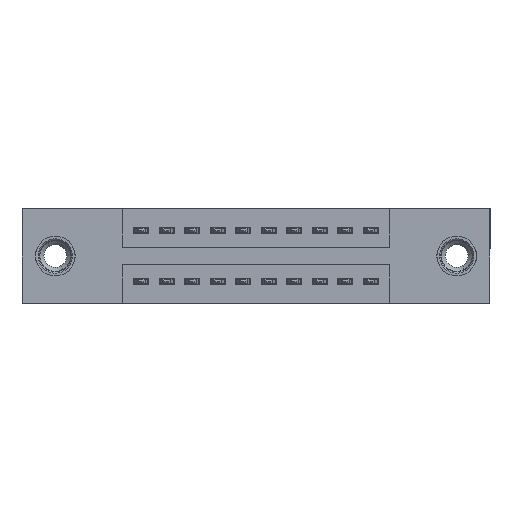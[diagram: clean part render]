
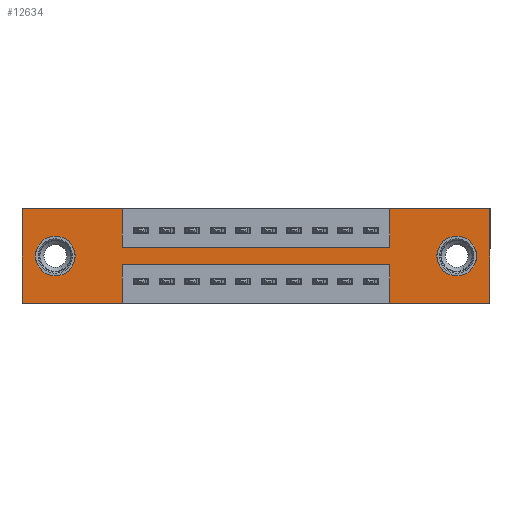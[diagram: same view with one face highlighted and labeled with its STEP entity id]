
A CAD part, front view. The second image highlights one B-rep face of the part: STEP entity #12634.
In plain terms, the highlighted planar face has unit normal (0, -1, 0).
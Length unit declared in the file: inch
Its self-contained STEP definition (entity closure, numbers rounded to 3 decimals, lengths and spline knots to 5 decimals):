
#121 = CARTESIAN_POINT ( 'NONE',  ( 0., 0., 0. ) ) ;
#182 = ORIENTED_EDGE ( 'NONE', *, *, #13849, .F. ) ;
#224 = CARTESIAN_POINT ( 'NONE',  ( 1.705, 0., -0.263 ) ) ;
#312 = LINE ( 'NONE', #5380, #14048 ) ;
#617 = EDGE_CURVE ( 'NONE', #8967, #3346, #3649, .T. ) ;
#716 = CIRCLE ( 'NONE', #15169, 0.078 ) ;
#773 = CARTESIAN_POINT ( 'NONE',  ( 0., 0., -0.37 ) ) ;
#866 = EDGE_CURVE ( 'NONE', #4796, #4143, #10822, .T. ) ;
#882 = DIRECTION ( 'NONE',  ( 1., 0., 0. ) ) ;
#990 = EDGE_CURVE ( 'NONE', #4143, #8967, #6941, .T. ) ;
#1279 = CARTESIAN_POINT ( 'NONE',  ( 0.3925, 0., 0. ) ) ;
#1297 = CARTESIAN_POINT ( 'NONE',  ( 0.3925, 0., -0.37 ) ) ;
#1778 = CARTESIAN_POINT ( 'NONE',  ( 1.4425, 0., -0.15 ) ) ;
#1867 = ORIENTED_EDGE ( 'NONE', *, *, #10916, .F. ) ;
#1991 = VERTEX_POINT ( 'NONE', #10762 ) ;
#1994 = DIRECTION ( 'NONE',  ( 0., 0., 1. ) ) ;
#2350 = CARTESIAN_POINT ( 'NONE',  ( 1.705, 0., -0.185 ) ) ;
#2549 = VERTEX_POINT ( 'NONE', #1279 ) ;
#2625 = CARTESIAN_POINT ( 'NONE',  ( 0., 0., 0. ) ) ;
#2673 = EDGE_CURVE ( 'NONE', #3155, #16917, #12116, .T. ) ;
#2813 = AXIS2_PLACEMENT_3D ( 'NONE', #13764, #5998, #15003 ) ;
#2911 = CIRCLE ( 'NONE', #12442, 0.078 ) ;
#3048 = CARTESIAN_POINT ( 'NONE',  ( 0.3925, 0., -0.22 ) ) ;
#3155 = VERTEX_POINT ( 'NONE', #12738 ) ;
#3212 = VECTOR ( 'NONE', #882, 39.37008 ) ;
#3346 = VERTEX_POINT ( 'NONE', #17023 ) ;
#3509 = CARTESIAN_POINT ( 'NONE',  ( 0.3925, 0., -0.15 ) ) ;
#3550 = ORIENTED_EDGE ( 'NONE', *, *, #15050, .F. ) ;
#3649 = LINE ( 'NONE', #121, #3212 ) ;
#3744 = CARTESIAN_POINT ( 'NONE',  ( 1.4425, 0., 0. ) ) ;
#3750 = DIRECTION ( 'NONE',  ( 0., 0., -1. ) ) ;
#3848 = VECTOR ( 'NONE', #6749, 39.37008 ) ;
#3890 = DIRECTION ( 'NONE',  ( 0., 0., 1. ) ) ;
#4140 = DIRECTION ( 'NONE',  ( 1., 0., 0. ) ) ;
#4143 = VERTEX_POINT ( 'NONE', #1778 ) ;
#4450 = VECTOR ( 'NONE', #16016, 39.37008 ) ;
#4638 = CARTESIAN_POINT ( 'NONE',  ( 1.4425, 0., 0. ) ) ;
#4796 = VERTEX_POINT ( 'NONE', #13777 ) ;
#4904 = VERTEX_POINT ( 'NONE', #12872 ) ;
#5045 = EDGE_CURVE ( 'NONE', #2549, #4796, #312, .T. ) ;
#5380 = CARTESIAN_POINT ( 'NONE',  ( 0.3925, 0., 0. ) ) ;
#5567 = ORIENTED_EDGE ( 'NONE', *, *, #12594, .T. ) ;
#5739 = VECTOR ( 'NONE', #14583, 39.37008 ) ;
#5972 = VERTEX_POINT ( 'NONE', #13733 ) ;
#5981 = CARTESIAN_POINT ( 'NONE',  ( 0., 0., -0.37 ) ) ;
#5998 = DIRECTION ( 'NONE',  ( 0., 1., 0. ) ) ;
#6016 = CARTESIAN_POINT ( 'NONE',  ( 1.4425, 0., -0.37 ) ) ;
#6048 = DIRECTION ( 'NONE',  ( 0., -1., 0. ) ) ;
#6098 = CARTESIAN_POINT ( 'NONE',  ( 0.13, 0., -0.263 ) ) ;
#6144 = CARTESIAN_POINT ( 'NONE',  ( 1.835, 0., 0. ) ) ;
#6189 = EDGE_CURVE ( 'NONE', #14736, #5972, #7317, .T. ) ;
#6308 = EDGE_LOOP ( 'NONE', ( #6847, #15502, #182, #16227, #7313, #9297, #8801, #12452, #8938, #3550, #16236, #1867 ) ) ;
#6440 = FACE_BOUND ( 'NONE', #16244, .T. ) ;
#6448 = EDGE_CURVE ( 'NONE', #7576, #1991, #716, .T. ) ;
#6749 = DIRECTION ( 'NONE',  ( 0., 0., -1. ) ) ;
#6782 = LINE ( 'NONE', #11856, #16581 ) ;
#6847 = ORIENTED_EDGE ( 'NONE', *, *, #6189, .F. ) ;
#6941 = LINE ( 'NONE', #3744, #5739 ) ;
#7313 = ORIENTED_EDGE ( 'NONE', *, *, #16451, .F. ) ;
#7314 = EDGE_CURVE ( 'NONE', #13949, #8840, #8773, .T. ) ;
#7317 = LINE ( 'NONE', #1297, #3848 ) ;
#7379 = CARTESIAN_POINT ( 'NONE',  ( 1.705, 0., -0.185 ) ) ;
#7576 = VERTEX_POINT ( 'NONE', #224 ) ;
#7912 = DIRECTION ( 'NONE',  ( 0., 0., 1. ) ) ;
#8158 = AXIS2_PLACEMENT_3D ( 'NONE', #8648, #6048, #15055 ) ;
#8265 = LINE ( 'NONE', #6016, #15074 ) ;
#8354 = CARTESIAN_POINT ( 'NONE',  ( 1.835, 0., -0.37 ) ) ;
#8471 = EDGE_CURVE ( 'NONE', #1991, #7576, #2911, .T. ) ;
#8606 = DIRECTION ( 'NONE',  ( 0., 1., 0. ) ) ;
#8648 = CARTESIAN_POINT ( 'NONE',  ( 0., 0., -0.37 ) ) ;
#8740 = DIRECTION ( 'NONE',  ( 0., 0., -1. ) ) ;
#8773 = LINE ( 'NONE', #2625, #12170 ) ;
#8801 = ORIENTED_EDGE ( 'NONE', *, *, #990, .F. ) ;
#8816 = DIRECTION ( 'NONE',  ( 0., 0., -1. ) ) ;
#8838 = DIRECTION ( 'NONE',  ( -1., 0., 0. ) ) ;
#8840 = VERTEX_POINT ( 'NONE', #10787 ) ;
#8846 = VECTOR ( 'NONE', #8816, 39.37008 ) ;
#8932 = CARTESIAN_POINT ( 'NONE',  ( 0.13, 0., -0.185 ) ) ;
#8938 = ORIENTED_EDGE ( 'NONE', *, *, #5045, .F. ) ;
#8967 = VERTEX_POINT ( 'NONE', #4638 ) ;
#9252 = LINE ( 'NONE', #6144, #8846 ) ;
#9297 = ORIENTED_EDGE ( 'NONE', *, *, #617, .F. ) ;
#9544 = FACE_OUTER_BOUND ( 'NONE', #6308, .T. ) ;
#9771 = ORIENTED_EDGE ( 'NONE', *, *, #8471, .T. ) ;
#9969 = PLANE ( 'NONE',  #8158 ) ;
#10200 = LINE ( 'NONE', #15160, #16111 ) ;
#10440 = VECTOR ( 'NONE', #4140, 39.37008 ) ;
#10638 = DIRECTION ( 'NONE',  ( 1., 0., 0. ) ) ;
#10762 = CARTESIAN_POINT ( 'NONE',  ( 1.705, 0., -0.107 ) ) ;
#10787 = CARTESIAN_POINT ( 'NONE',  ( 0., 0., 0. ) ) ;
#10822 = LINE ( 'NONE', #3509, #10440 ) ;
#10835 = LINE ( 'NONE', #5981, #13466 ) ;
#10916 = EDGE_CURVE ( 'NONE', #5972, #13949, #10200, .T. ) ;
#11051 = CARTESIAN_POINT ( 'NONE',  ( 0.3925, 0., -0.22 ) ) ;
#11250 = CARTESIAN_POINT ( 'NONE',  ( 1.4425, 0., -0.37 ) ) ;
#11328 = EDGE_CURVE ( 'NONE', #4904, #14736, #14363, .T. ) ;
#11332 = AXIS2_PLACEMENT_3D ( 'NONE', #8932, #8606, #3890 ) ;
#11593 = DIRECTION ( 'NONE',  ( 0., 1., 0. ) ) ;
#11856 = CARTESIAN_POINT ( 'NONE',  ( 0., 0., 0. ) ) ;
#12116 = CIRCLE ( 'NONE', #11332, 0.078 ) ;
#12170 = VECTOR ( 'NONE', #7912, 39.37008 ) ;
#12442 = AXIS2_PLACEMENT_3D ( 'NONE', #2350, #11593, #3750 ) ;
#12452 = ORIENTED_EDGE ( 'NONE', *, *, #866, .F. ) ;
#12594 = EDGE_CURVE ( 'NONE', #16917, #3155, #16262, .T. ) ;
#12634 = ADVANCED_FACE ( 'NONE', ( #6440, #15870, #9544 ), #9969, .T. ) ;
#12738 = CARTESIAN_POINT ( 'NONE',  ( 0.13, 0., -0.107 ) ) ;
#12872 = CARTESIAN_POINT ( 'NONE',  ( 1.4425, 0., -0.22 ) ) ;
#13466 = VECTOR ( 'NONE', #14983, 39.37008 ) ;
#13597 = ORIENTED_EDGE ( 'NONE', *, *, #2673, .T. ) ;
#13733 = CARTESIAN_POINT ( 'NONE',  ( 0.3925, 0., -0.37 ) ) ;
#13764 = CARTESIAN_POINT ( 'NONE',  ( 0.13, 0., -0.185 ) ) ;
#13777 = CARTESIAN_POINT ( 'NONE',  ( 0.3925, 0., -0.15 ) ) ;
#13849 = EDGE_CURVE ( 'NONE', #14387, #4904, #8265, .T. ) ;
#13949 = VERTEX_POINT ( 'NONE', #773 ) ;
#14048 = VECTOR ( 'NONE', #16884, 39.37008 ) ;
#14363 = LINE ( 'NONE', #3048, #4450 ) ;
#14387 = VERTEX_POINT ( 'NONE', #11250 ) ;
#14497 = ORIENTED_EDGE ( 'NONE', *, *, #6448, .T. ) ;
#14583 = DIRECTION ( 'NONE',  ( 0., 0., 1. ) ) ;
#14736 = VERTEX_POINT ( 'NONE', #11051 ) ;
#14983 = DIRECTION ( 'NONE',  ( -1., 0., 0. ) ) ;
#15003 = DIRECTION ( 'NONE',  ( 0., 0., 1. ) ) ;
#15050 = EDGE_CURVE ( 'NONE', #8840, #2549, #6782, .T. ) ;
#15055 = DIRECTION ( 'NONE',  ( 0., 0., -1. ) ) ;
#15074 = VECTOR ( 'NONE', #1994, 39.37008 ) ;
#15147 = VERTEX_POINT ( 'NONE', #8354 ) ;
#15160 = CARTESIAN_POINT ( 'NONE',  ( 0., 0., -0.37 ) ) ;
#15169 = AXIS2_PLACEMENT_3D ( 'NONE', #7379, #16328, #8740 ) ;
#15502 = ORIENTED_EDGE ( 'NONE', *, *, #11328, .F. ) ;
#15870 = FACE_BOUND ( 'NONE', #16928, .T. ) ;
#16016 = DIRECTION ( 'NONE',  ( -1., 0., 0. ) ) ;
#16111 = VECTOR ( 'NONE', #8838, 39.37008 ) ;
#16227 = ORIENTED_EDGE ( 'NONE', *, *, #16385, .F. ) ;
#16236 = ORIENTED_EDGE ( 'NONE', *, *, #7314, .F. ) ;
#16244 = EDGE_LOOP ( 'NONE', ( #9771, #14497 ) ) ;
#16262 = CIRCLE ( 'NONE', #2813, 0.078 ) ;
#16328 = DIRECTION ( 'NONE',  ( 0., 1., 0. ) ) ;
#16385 = EDGE_CURVE ( 'NONE', #15147, #14387, #10835, .T. ) ;
#16451 = EDGE_CURVE ( 'NONE', #3346, #15147, #9252, .T. ) ;
#16581 = VECTOR ( 'NONE', #10638, 39.37008 ) ;
#16884 = DIRECTION ( 'NONE',  ( 0., 0., -1. ) ) ;
#16917 = VERTEX_POINT ( 'NONE', #6098 ) ;
#16928 = EDGE_LOOP ( 'NONE', ( #13597, #5567 ) ) ;
#17023 = CARTESIAN_POINT ( 'NONE',  ( 1.835, 0., 0. ) ) ;
